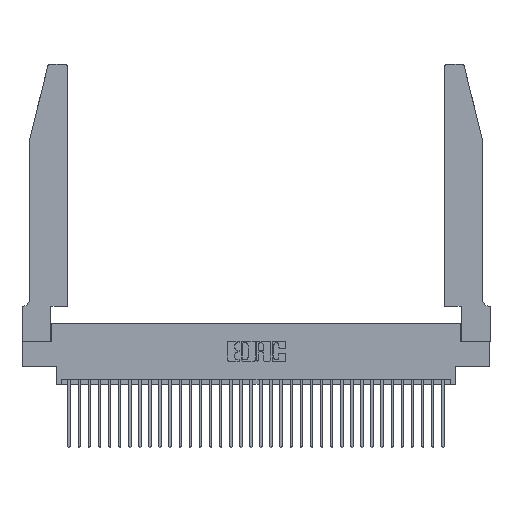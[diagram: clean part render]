
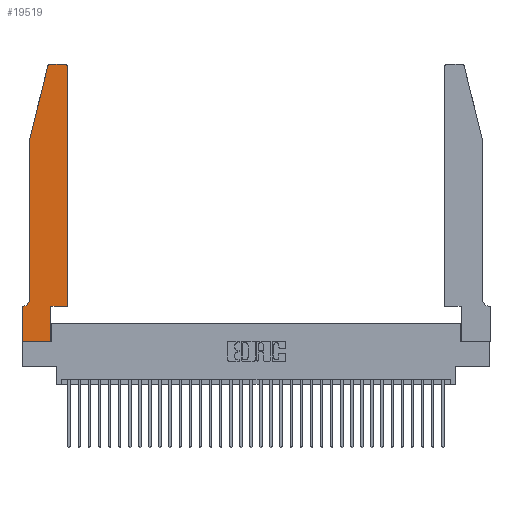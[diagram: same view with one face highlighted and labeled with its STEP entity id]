
A CAD part, top view. The second image highlights one B-rep face of the part: STEP entity #19519.
In plain terms, the highlighted planar face has unit normal (0, 0, 1).
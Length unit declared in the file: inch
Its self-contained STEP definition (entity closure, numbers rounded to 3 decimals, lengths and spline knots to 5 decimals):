
#232 = EDGE_CURVE ( 'NONE', #22650, #555, #23911, .T. ) ;
#434 = FACE_OUTER_BOUND ( 'NONE', #29466, .T. ) ;
#555 = VERTEX_POINT ( 'NONE', #33981 ) ;
#980 = AXIS2_PLACEMENT_3D ( 'NONE', #3841, #21944, #18680 ) ;
#1153 = DIRECTION ( 'NONE',  ( 1., 0., 0. ) ) ;
#2009 = VECTOR ( 'NONE', #18038, 39.37008 ) ;
#2862 = CARTESIAN_POINT ( 'NONE',  ( 0.2865, 0.35, 0.37 ) ) ;
#3681 = LINE ( 'NONE', #31810, #27548 ) ;
#3841 = CARTESIAN_POINT ( 'NONE',  ( 0., 0.35, 0.37 ) ) ;
#4015 = VECTOR ( 'NONE', #29743, 39.37008 ) ;
#4161 = VECTOR ( 'NONE', #11594, 39.37008 ) ;
#4278 = CARTESIAN_POINT ( 'NONE',  ( 0.4205, 2.75, 0.37 ) ) ;
#4471 = LINE ( 'NONE', #21590, #13008 ) ;
#4568 = EDGE_CURVE ( 'NONE', #13733, #34605, #16778, .T. ) ;
#5287 = VERTEX_POINT ( 'NONE', #15710 ) ;
#5659 = ORIENTED_EDGE ( 'NONE', *, *, #21030, .T. ) ;
#6423 = EDGE_CURVE ( 'NONE', #26149, #22650, #4471, .T. ) ;
#7438 = CARTESIAN_POINT ( 'NONE',  ( 0., 0.35, 0.37 ) ) ;
#8427 = DIRECTION ( 'NONE',  ( -1., 0., 0. ) ) ;
#8586 = CARTESIAN_POINT ( 'NONE',  ( 0.4505, 0.35, 0.37 ) ) ;
#8664 = ORIENTED_EDGE ( 'NONE', *, *, #35101, .T. ) ;
#9571 = AXIS2_PLACEMENT_3D ( 'NONE', #30688, #14639, #1153 ) ;
#9642 = CARTESIAN_POINT ( 'NONE',  ( 0.0055, 0.42, 0.37 ) ) ;
#9942 = LINE ( 'NONE', #19230, #17532 ) ;
#11026 = DIRECTION ( 'NONE',  ( 1., 0., 0. ) ) ;
#11103 = CARTESIAN_POINT ( 'NONE',  ( 0.25487, 2.72718, 0.37 ) ) ;
#11594 = DIRECTION ( 'NONE',  ( 0., -1., 0. ) ) ;
#11642 = DIRECTION ( 'NONE',  ( 0., 1., 0. ) ) ;
#11818 = CARTESIAN_POINT ( 'NONE',  ( 0., 0., 0.37 ) ) ;
#12098 = LINE ( 'NONE', #2862, #34228 ) ;
#12484 = CIRCLE ( 'NONE', #19086, 0.03 ) ;
#12870 = CARTESIAN_POINT ( 'NONE',  ( 0.0755, 2., 0.37 ) ) ;
#13008 = VECTOR ( 'NONE', #11026, 39.37008 ) ;
#13355 = CARTESIAN_POINT ( 'NONE',  ( 0.0755, 0.35, 0.37 ) ) ;
#13733 = VERTEX_POINT ( 'NONE', #33957 ) ;
#14029 = EDGE_CURVE ( 'NONE', #32936, #19303, #9942, .T. ) ;
#14110 = CARTESIAN_POINT ( 'NONE',  ( 0.284, 2.75, 0.37 ) ) ;
#14127 = EDGE_CURVE ( 'NONE', #555, #21738, #14614, .T. ) ;
#14428 = EDGE_CURVE ( 'NONE', #34239, #32936, #12484, .T. ) ;
#14605 = PLANE ( 'NONE',  #980 ) ;
#14614 = CIRCLE ( 'NONE', #9571, 0.03 ) ;
#14639 = DIRECTION ( 'NONE',  ( 0., 0., 1. ) ) ;
#15175 = VERTEX_POINT ( 'NONE', #32621 ) ;
#15196 = ORIENTED_EDGE ( 'NONE', *, *, #4568, .T. ) ;
#15710 = CARTESIAN_POINT ( 'NONE',  ( 0.2865, 0., 0.37 ) ) ;
#16778 = LINE ( 'NONE', #13355, #4015 ) ;
#16805 = ORIENTED_EDGE ( 'NONE', *, *, #14127, .T. ) ;
#16923 = CARTESIAN_POINT ( 'NONE',  ( 0.0755, 0.42, 0.37 ) ) ;
#17532 = VECTOR ( 'NONE', #27455, 39.37008 ) ;
#17680 = DIRECTION ( 'NONE',  ( -1., 0., 0. ) ) ;
#17734 = DIRECTION ( 'NONE',  ( 1., 0., 0. ) ) ;
#17793 = DIRECTION ( 'NONE',  ( 0., 0., -1. ) ) ;
#18038 = DIRECTION ( 'NONE',  ( 0., -1., 0. ) ) ;
#18680 = DIRECTION ( 'NONE',  ( 1., 0., 0. ) ) ;
#19086 = AXIS2_PLACEMENT_3D ( 'NONE', #27750, #33380, #17734 ) ;
#19230 = CARTESIAN_POINT ( 'NONE',  ( 0.0755, 2., 0.37 ) ) ;
#19303 = VERTEX_POINT ( 'NONE', #20539 ) ;
#19519 = ADVANCED_FACE ( 'NONE', ( #434 ), #14605, .T. ) ;
#20539 = CARTESIAN_POINT ( 'NONE',  ( 0.0755, 2., 0.37 ) ) ;
#21030 = EDGE_CURVE ( 'NONE', #21738, #34239, #25843, .T. ) ;
#21130 = EDGE_CURVE ( 'NONE', #15175, #5287, #3681, .T. ) ;
#21590 = CARTESIAN_POINT ( 'NONE',  ( 0.4505, 0.35, 0.37 ) ) ;
#21738 = VERTEX_POINT ( 'NONE', #4278 ) ;
#21910 = DIRECTION ( 'NONE',  ( 0., 1., 0. ) ) ;
#21944 = DIRECTION ( 'NONE',  ( 0., 0., 1. ) ) ;
#22070 = LINE ( 'NONE', #11818, #4161 ) ;
#22631 = VECTOR ( 'NONE', #11642, 39.37008 ) ;
#22650 = VERTEX_POINT ( 'NONE', #8586 ) ;
#23128 = ORIENTED_EDGE ( 'NONE', *, *, #14428, .T. ) ;
#23911 = LINE ( 'NONE', #28143, #22631 ) ;
#24338 = EDGE_CURVE ( 'NONE', #25670, #13733, #29470, .T. ) ;
#24722 = CARTESIAN_POINT ( 'NONE',  ( 0.2605, 2.75, 0.37 ) ) ;
#24824 = ORIENTED_EDGE ( 'NONE', *, *, #232, .T. ) ;
#25670 = VERTEX_POINT ( 'NONE', #16923 ) ;
#25843 = LINE ( 'NONE', #24722, #28398 ) ;
#25859 = ORIENTED_EDGE ( 'NONE', *, *, #14029, .T. ) ;
#26149 = VERTEX_POINT ( 'NONE', #35145 ) ;
#27205 = EDGE_CURVE ( 'NONE', #34605, #15175, #22070, .T. ) ;
#27420 = ORIENTED_EDGE ( 'NONE', *, *, #6423, .T. ) ;
#27448 = ORIENTED_EDGE ( 'NONE', *, *, #30735, .T. ) ;
#27455 = DIRECTION ( 'NONE',  ( -0.239, -0.971, 0. ) ) ;
#27548 = VECTOR ( 'NONE', #34103, 39.37008 ) ;
#27750 = CARTESIAN_POINT ( 'NONE',  ( 0.284, 2.72, 0.37 ) ) ;
#27968 = LINE ( 'NONE', #12870, #2009 ) ;
#28143 = CARTESIAN_POINT ( 'NONE',  ( 0.4505, 0.35, 0.37 ) ) ;
#28398 = VECTOR ( 'NONE', #8427, 39.37008 ) ;
#28552 = ORIENTED_EDGE ( 'NONE', *, *, #21130, .T. ) ;
#29466 = EDGE_LOOP ( 'NONE', ( #5659, #23128, #25859, #8664, #32473, #15196, #34034, #28552, #27448, #27420, #24824, #16805 ) ) ;
#29470 = CIRCLE ( 'NONE', #34865, 0.07 ) ;
#29743 = DIRECTION ( 'NONE',  ( -1., 0., 0. ) ) ;
#30688 = CARTESIAN_POINT ( 'NONE',  ( 0.4205, 2.72, 0.37 ) ) ;
#30735 = EDGE_CURVE ( 'NONE', #5287, #26149, #12098, .T. ) ;
#31810 = CARTESIAN_POINT ( 'NONE',  ( 0., 0., 0.37 ) ) ;
#32473 = ORIENTED_EDGE ( 'NONE', *, *, #24338, .T. ) ;
#32621 = CARTESIAN_POINT ( 'NONE',  ( 0., 0., 0.37 ) ) ;
#32936 = VERTEX_POINT ( 'NONE', #11103 ) ;
#33380 = DIRECTION ( 'NONE',  ( 0., 0., 1. ) ) ;
#33957 = CARTESIAN_POINT ( 'NONE',  ( 0.0055, 0.35, 0.37 ) ) ;
#33981 = CARTESIAN_POINT ( 'NONE',  ( 0.4505, 2.72, 0.37 ) ) ;
#34034 = ORIENTED_EDGE ( 'NONE', *, *, #27205, .T. ) ;
#34103 = DIRECTION ( 'NONE',  ( 1., 0., 0. ) ) ;
#34228 = VECTOR ( 'NONE', #21910, 39.37008 ) ;
#34239 = VERTEX_POINT ( 'NONE', #14110 ) ;
#34605 = VERTEX_POINT ( 'NONE', #7438 ) ;
#34865 = AXIS2_PLACEMENT_3D ( 'NONE', #9642, #17793, #17680 ) ;
#35101 = EDGE_CURVE ( 'NONE', #19303, #25670, #27968, .T. ) ;
#35145 = CARTESIAN_POINT ( 'NONE',  ( 0.2865, 0.35, 0.37 ) ) ;
